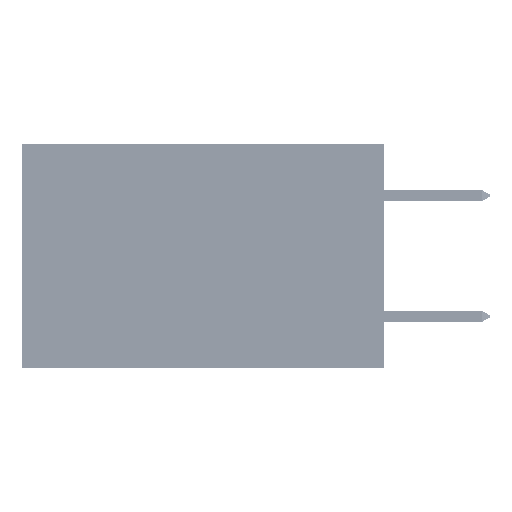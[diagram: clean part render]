
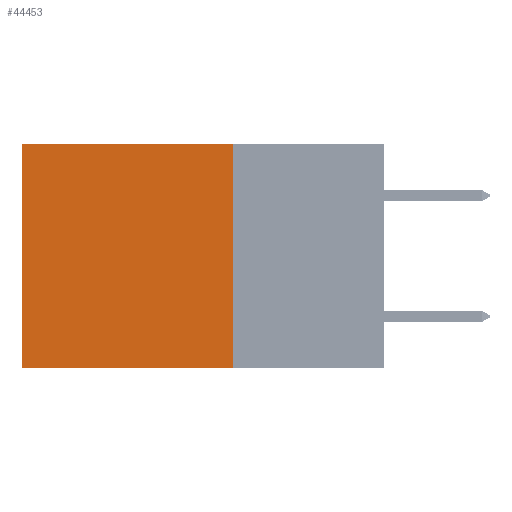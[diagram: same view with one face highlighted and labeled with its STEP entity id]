
A CAD part, left-side view. The second image highlights one B-rep face of the part: STEP entity #44453.
In plain terms, the highlighted planar face has unit normal (-1, 0, 0).
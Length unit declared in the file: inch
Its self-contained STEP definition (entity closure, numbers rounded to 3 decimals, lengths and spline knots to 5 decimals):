
#321 = ORIENTED_EDGE ( 'NONE', *, *, #18971, .T. ) ;
#1330 = FACE_OUTER_BOUND ( 'NONE', #43791, .T. ) ;
#2869 = DIRECTION ( 'NONE',  ( 0., 0., -1. ) ) ;
#3782 = AXIS2_PLACEMENT_3D ( 'NONE', #33836, #49775, #17354 ) ;
#4673 = CARTESIAN_POINT ( 'NONE',  ( 0.2875, 0.6, 0. ) ) ;
#5000 = DIRECTION ( 'NONE',  ( 0., 0., -1. ) ) ;
#6778 = VERTEX_POINT ( 'NONE', #25350 ) ;
#7141 = VECTOR ( 'NONE', #5000, 39.37008 ) ;
#7450 = CARTESIAN_POINT ( 'NONE',  ( 0.2875, 0.6, -0.37 ) ) ;
#7607 = LINE ( 'NONE', #43777, #7658 ) ;
#7658 = VECTOR ( 'NONE', #11529, 39.37008 ) ;
#9129 = CARTESIAN_POINT ( 'NONE',  ( 0.2875, 0.25, 0. ) ) ;
#9182 = CARTESIAN_POINT ( 'NONE',  ( 0.2875, 0.25, 0. ) ) ;
#10455 = VERTEX_POINT ( 'NONE', #9129 ) ;
#11529 = DIRECTION ( 'NONE',  ( 0., 1., 0. ) ) ;
#13266 = VERTEX_POINT ( 'NONE', #4673 ) ;
#14104 = ORIENTED_EDGE ( 'NONE', *, *, #50391, .T. ) ;
#14214 = CARTESIAN_POINT ( 'NONE',  ( 0.2875, 0.25, 0. ) ) ;
#15916 = VECTOR ( 'NONE', #17387, 39.37008 ) ;
#16110 = ORIENTED_EDGE ( 'NONE', *, *, #35973, .F. ) ;
#17354 = DIRECTION ( 'NONE',  ( 0., 0., -1. ) ) ;
#17387 = DIRECTION ( 'NONE',  ( 0., 1., 0. ) ) ;
#18971 = EDGE_CURVE ( 'NONE', #13266, #39669, #39026, .T. ) ;
#21281 = PLANE ( 'NONE',  #3782 ) ;
#24029 = EDGE_CURVE ( 'NONE', #10455, #6778, #29645, .T. ) ;
#24412 = ORIENTED_EDGE ( 'NONE', *, *, #24029, .F. ) ;
#25350 = CARTESIAN_POINT ( 'NONE',  ( 0.2875, 0.25, -0.37 ) ) ;
#27162 = VECTOR ( 'NONE', #2869, 39.37008 ) ;
#29645 = LINE ( 'NONE', #9182, #7141 ) ;
#30913 = CARTESIAN_POINT ( 'NONE',  ( 0.2875, 0.6, 0. ) ) ;
#33836 = CARTESIAN_POINT ( 'NONE',  ( 0.2875, 0.25, 0. ) ) ;
#35973 = EDGE_CURVE ( 'NONE', #6778, #39669, #7607, .T. ) ;
#39026 = LINE ( 'NONE', #30913, #27162 ) ;
#39669 = VERTEX_POINT ( 'NONE', #7450 ) ;
#43777 = CARTESIAN_POINT ( 'NONE',  ( 0.2875, 0.25, -0.37 ) ) ;
#43791 = EDGE_LOOP ( 'NONE', ( #321, #16110, #24412, #14104 ) ) ;
#44453 = ADVANCED_FACE ( 'NONE', ( #1330 ), #21281, .F. ) ;
#49775 = DIRECTION ( 'NONE',  ( 1., 0., 0. ) ) ;
#50074 = LINE ( 'NONE', #14214, #15916 ) ;
#50391 = EDGE_CURVE ( 'NONE', #10455, #13266, #50074, .T. ) ;
